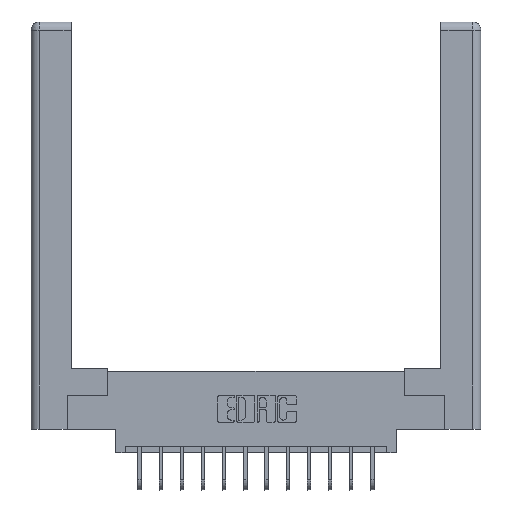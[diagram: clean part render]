
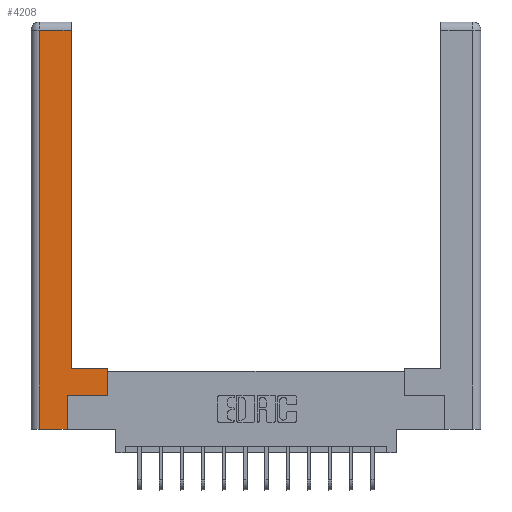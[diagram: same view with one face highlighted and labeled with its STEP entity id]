
A CAD part, top view. The second image highlights one B-rep face of the part: STEP entity #4208.
In plain terms, the highlighted planar face has unit normal (0, 0, 1).
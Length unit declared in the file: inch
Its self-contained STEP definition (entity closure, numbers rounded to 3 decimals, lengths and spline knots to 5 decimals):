
#108 = VECTOR ( 'NONE', #4763, 39.37008 ) ;
#244 = ORIENTED_EDGE ( 'NONE', *, *, #9487, .T. ) ;
#277 = VECTOR ( 'NONE', #6775, 39.37008 ) ;
#422 = VECTOR ( 'NONE', #17712, 39.37008 ) ;
#573 = EDGE_LOOP ( 'NONE', ( #13876, #10852, #11909, #1462, #13200, #6199, #244, #13394 ) ) ;
#739 = LINE ( 'NONE', #4185, #2037 ) ;
#803 = CARTESIAN_POINT ( 'NONE',  ( 0.265, 0., 0. ) ) ;
#1267 = EDGE_CURVE ( 'NONE', #5021, #15215, #14327, .T. ) ;
#1293 = CARTESIAN_POINT ( 'NONE',  ( 0.295, 2.94, 0. ) ) ;
#1337 = CARTESIAN_POINT ( 'NONE',  ( 0.0615, 2.94, 0. ) ) ;
#1462 = ORIENTED_EDGE ( 'NONE', *, *, #17252, .T. ) ;
#1499 = LINE ( 'NONE', #8005, #14638 ) ;
#1638 = CARTESIAN_POINT ( 'NONE',  ( 0., 0., 0. ) ) ;
#1654 = DIRECTION ( 'NONE',  ( 1., 0., 0. ) ) ;
#1965 = VERTEX_POINT ( 'NONE', #14483 ) ;
#2037 = VECTOR ( 'NONE', #1654, 39.37008 ) ;
#2847 = VERTEX_POINT ( 'NONE', #9313 ) ;
#2915 = PLANE ( 'NONE',  #9925 ) ;
#3263 = FACE_OUTER_BOUND ( 'NONE', #573, .T. ) ;
#3561 = CARTESIAN_POINT ( 'NONE',  ( 0.265, 0.245, 0. ) ) ;
#4185 = CARTESIAN_POINT ( 'NONE',  ( 0.265, 0., 0. ) ) ;
#4208 = ADVANCED_FACE ( 'NONE', ( #3263 ), #2915, .F. ) ;
#4364 = CARTESIAN_POINT ( 'NONE',  ( 0.565, 0.245, 0. ) ) ;
#4613 = VERTEX_POINT ( 'NONE', #11700 ) ;
#4763 = DIRECTION ( 'NONE',  ( 0., 1., 0. ) ) ;
#5021 = VERTEX_POINT ( 'NONE', #803 ) ;
#5086 = VECTOR ( 'NONE', #10101, 39.37008 ) ;
#5246 = DIRECTION ( 'NONE',  ( 0., -1., 0. ) ) ;
#5284 = EDGE_CURVE ( 'NONE', #7235, #7475, #11250, .T. ) ;
#5352 = CARTESIAN_POINT ( 'NONE',  ( 0.295, 3., 0. ) ) ;
#6159 = CARTESIAN_POINT ( 'NONE',  ( 0.265, 0.245, 0. ) ) ;
#6199 = ORIENTED_EDGE ( 'NONE', *, *, #17257, .T. ) ;
#6241 = CARTESIAN_POINT ( 'NONE',  ( 0.295, 0.45, 0. ) ) ;
#6546 = LINE ( 'NONE', #4364, #15141 ) ;
#6775 = DIRECTION ( 'NONE',  ( 0., 1., 0. ) ) ;
#6835 = EDGE_CURVE ( 'NONE', #1965, #7949, #1499, .T. ) ;
#7235 = VERTEX_POINT ( 'NONE', #6241 ) ;
#7475 = VERTEX_POINT ( 'NONE', #1293 ) ;
#7479 = VECTOR ( 'NONE', #15361, 39.37008 ) ;
#7949 = VERTEX_POINT ( 'NONE', #9220 ) ;
#8005 = CARTESIAN_POINT ( 'NONE',  ( 0.0615, 0., 0. ) ) ;
#9220 = CARTESIAN_POINT ( 'NONE',  ( 0.0615, 0., 0. ) ) ;
#9241 = LINE ( 'NONE', #1337, #422 ) ;
#9313 = CARTESIAN_POINT ( 'NONE',  ( 0.565, 0.245, 0. ) ) ;
#9487 = EDGE_CURVE ( 'NONE', #2847, #4613, #17292, .T. ) ;
#9925 = AXIS2_PLACEMENT_3D ( 'NONE', #1638, #16865, #16685 ) ;
#10068 = LINE ( 'NONE', #16732, #7479 ) ;
#10101 = DIRECTION ( 'NONE',  ( 0., 1., 0. ) ) ;
#10852 = ORIENTED_EDGE ( 'NONE', *, *, #12093, .T. ) ;
#11250 = LINE ( 'NONE', #5352, #277 ) ;
#11700 = CARTESIAN_POINT ( 'NONE',  ( 0.565, 0.45, 0. ) ) ;
#11909 = ORIENTED_EDGE ( 'NONE', *, *, #6835, .T. ) ;
#12093 = EDGE_CURVE ( 'NONE', #7475, #1965, #9241, .T. ) ;
#13200 = ORIENTED_EDGE ( 'NONE', *, *, #1267, .T. ) ;
#13394 = ORIENTED_EDGE ( 'NONE', *, *, #16795, .T. ) ;
#13876 = ORIENTED_EDGE ( 'NONE', *, *, #5284, .T. ) ;
#14327 = LINE ( 'NONE', #6159, #5086 ) ;
#14483 = CARTESIAN_POINT ( 'NONE',  ( 0.0615, 2.94, 0. ) ) ;
#14638 = VECTOR ( 'NONE', #5246, 39.37008 ) ;
#15141 = VECTOR ( 'NONE', #15220, 39.37008 ) ;
#15215 = VERTEX_POINT ( 'NONE', #3561 ) ;
#15220 = DIRECTION ( 'NONE',  ( 1., 0., 0. ) ) ;
#15361 = DIRECTION ( 'NONE',  ( -1., 0., 0. ) ) ;
#15763 = CARTESIAN_POINT ( 'NONE',  ( 0.565, 0.45, 0. ) ) ;
#16685 = DIRECTION ( 'NONE',  ( -1., 0., 0. ) ) ;
#16732 = CARTESIAN_POINT ( 'NONE',  ( 0.295, 0.45, 0. ) ) ;
#16795 = EDGE_CURVE ( 'NONE', #4613, #7235, #10068, .T. ) ;
#16865 = DIRECTION ( 'NONE',  ( 0., 0., -1. ) ) ;
#17252 = EDGE_CURVE ( 'NONE', #7949, #5021, #739, .T. ) ;
#17257 = EDGE_CURVE ( 'NONE', #15215, #2847, #6546, .T. ) ;
#17292 = LINE ( 'NONE', #15763, #108 ) ;
#17712 = DIRECTION ( 'NONE',  ( -1., 0., 0. ) ) ;
